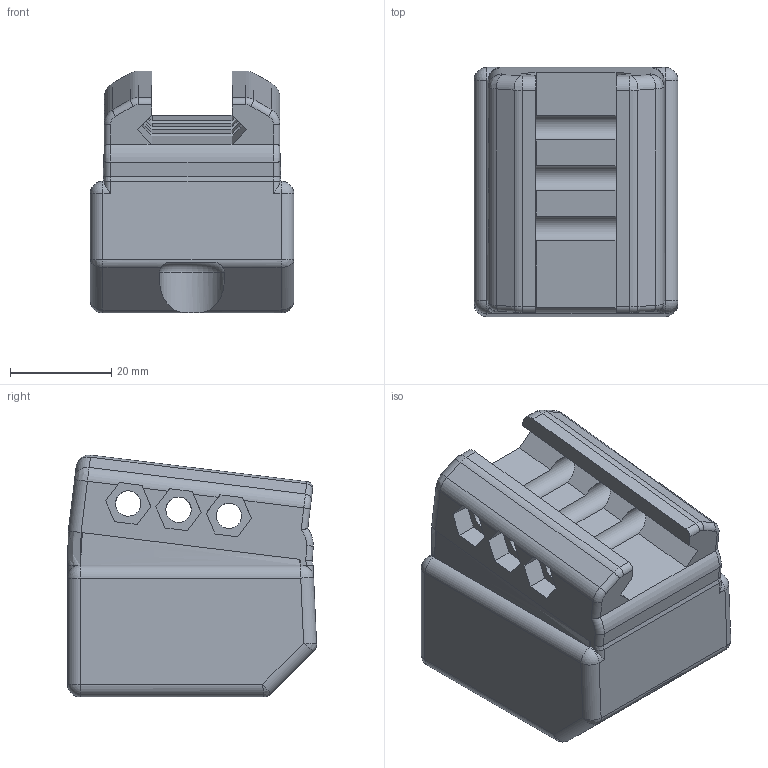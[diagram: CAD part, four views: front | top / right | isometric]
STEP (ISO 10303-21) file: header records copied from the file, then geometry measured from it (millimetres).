
FILE_DESCRIPTION(/* description */ (''),/* implementation_level */ '2;1');
FILE_NAME(/* name */ 'AR15 Buffer Tube Adapter - Dropped End.stp',/* time_stamp */ '2021-10-31T22:53:28-05:00',/* author */ ('johne'),/* organization */ (''),/* preprocessor_version */ 'ST-DEVELOPER v18.1',/* originating_system */ 'Autodesk Inventor 2020',/* authorisation */ '');
FILE_SCHEMA (('AUTOMOTIVE_DESIGN { 1 0 10303 214 3 1 1 }'));
Length unit declared in the file: inch
Products named in the file (1): AR15 Buffer Tube Adapter - Dropped End
Bounding box: 40.2 x 49.14 x 47.74 mm (x, y, z)
Volume: 57590.4 mm3; surface area: 15055.4 mm2
Topology: 1 solids, 1 shells, 161 faces, 424 edges, 256 vertices
Faces by surface type: plane 69, cylinder 56, bspline 22, torus 7, sphere 6, cone 1
Full cylindrical faces by diameter (mm): 5 x3, 29.808 x8
Entity records: 11806 total; most frequent: CARTESIAN_POINT 7875, ORIENTED_EDGE 840, DIRECTION 787, EDGE_CURVE 420, AXIS2_PLACEMENT_3D 280, VERTEX_POINT 256, LINE 227, VECTOR 227
